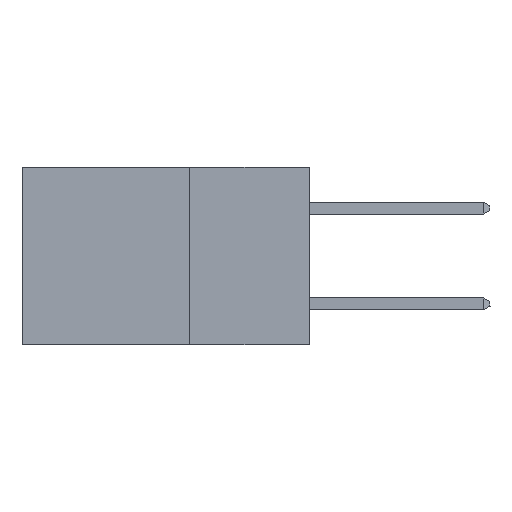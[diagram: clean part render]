
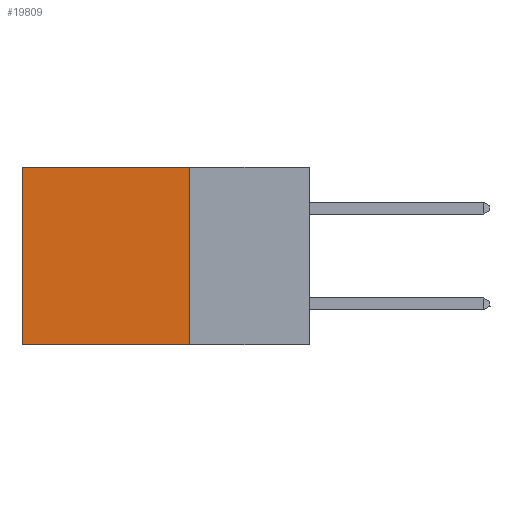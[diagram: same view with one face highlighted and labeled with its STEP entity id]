
A CAD part, left-side view. The second image highlights one B-rep face of the part: STEP entity #19809.
In plain terms, the highlighted planar face has unit normal (-1, 0, 0).
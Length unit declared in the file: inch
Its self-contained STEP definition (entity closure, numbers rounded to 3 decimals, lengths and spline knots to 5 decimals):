
#650 = LINE ( 'NONE', #15324, #10620 ) ;
#2144 = LINE ( 'NONE', #7359, #4325 ) ;
#2530 = VECTOR ( 'NONE', #21109, 39.37008 ) ;
#2670 = VERTEX_POINT ( 'NONE', #15277 ) ;
#2949 = CARTESIAN_POINT ( 'NONE',  ( 0.2875, 0.6, 0. ) ) ;
#3067 = CARTESIAN_POINT ( 'NONE',  ( 0.2875, 0.25, -0.37 ) ) ;
#3706 = VERTEX_POINT ( 'NONE', #3067 ) ;
#4325 = VECTOR ( 'NONE', #23640, 39.37008 ) ;
#5157 = ORIENTED_EDGE ( 'NONE', *, *, #18728, .F. ) ;
#5335 = LINE ( 'NONE', #15946, #2530 ) ;
#5857 = CARTESIAN_POINT ( 'NONE',  ( 0.2875, 0.25, 0. ) ) ;
#5905 = CARTESIAN_POINT ( 'NONE',  ( 0.2875, 0.25, 0. ) ) ;
#6937 = DIRECTION ( 'NONE',  ( 0., 1., 0. ) ) ;
#7359 = CARTESIAN_POINT ( 'NONE',  ( 0.2875, 0.25, -0.37 ) ) ;
#7862 = DIRECTION ( 'NONE',  ( 0., 0., -1. ) ) ;
#7994 = EDGE_LOOP ( 'NONE', ( #24758, #21308, #5157, #17043 ) ) ;
#8001 = LINE ( 'NONE', #5905, #11395 ) ;
#8299 = EDGE_CURVE ( 'NONE', #20692, #21045, #5335, .T. ) ;
#10620 = VECTOR ( 'NONE', #23408, 39.37008 ) ;
#11395 = VECTOR ( 'NONE', #6937, 39.37008 ) ;
#13961 = FACE_OUTER_BOUND ( 'NONE', #7994, .T. ) ;
#15214 = EDGE_CURVE ( 'NONE', #3706, #21045, #2144, .T. ) ;
#15277 = CARTESIAN_POINT ( 'NONE',  ( 0.2875, 0.25, 0. ) ) ;
#15324 = CARTESIAN_POINT ( 'NONE',  ( 0.2875, 0.25, 0. ) ) ;
#15854 = AXIS2_PLACEMENT_3D ( 'NONE', #5857, #19710, #7862 ) ;
#15946 = CARTESIAN_POINT ( 'NONE',  ( 0.2875, 0.6, 0. ) ) ;
#17043 = ORIENTED_EDGE ( 'NONE', *, *, #21522, .T. ) ;
#18728 = EDGE_CURVE ( 'NONE', #2670, #3706, #650, .T. ) ;
#19193 = PLANE ( 'NONE',  #15854 ) ;
#19710 = DIRECTION ( 'NONE',  ( 1., 0., 0. ) ) ;
#19809 = ADVANCED_FACE ( 'NONE', ( #13961 ), #19193, .F. ) ;
#20692 = VERTEX_POINT ( 'NONE', #2949 ) ;
#21045 = VERTEX_POINT ( 'NONE', #25650 ) ;
#21109 = DIRECTION ( 'NONE',  ( 0., 0., -1. ) ) ;
#21308 = ORIENTED_EDGE ( 'NONE', *, *, #15214, .F. ) ;
#21522 = EDGE_CURVE ( 'NONE', #2670, #20692, #8001, .T. ) ;
#23408 = DIRECTION ( 'NONE',  ( 0., 0., -1. ) ) ;
#23640 = DIRECTION ( 'NONE',  ( 0., 1., 0. ) ) ;
#24758 = ORIENTED_EDGE ( 'NONE', *, *, #8299, .T. ) ;
#25650 = CARTESIAN_POINT ( 'NONE',  ( 0.2875, 0.6, -0.37 ) ) ;
